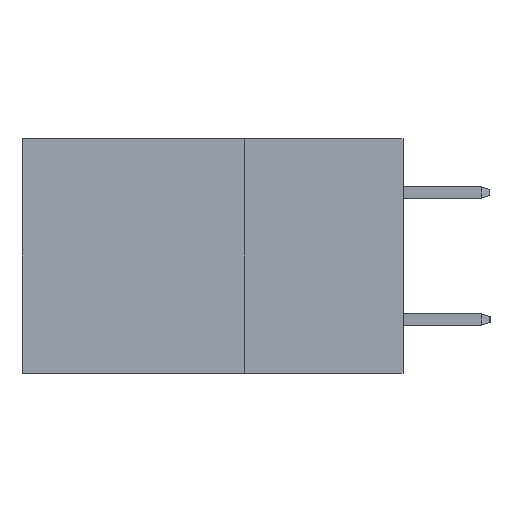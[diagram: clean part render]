
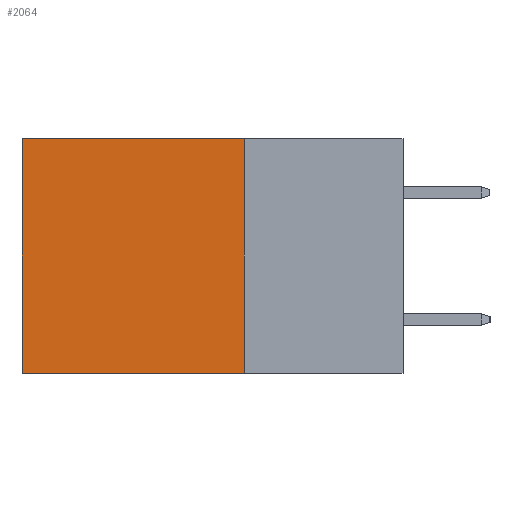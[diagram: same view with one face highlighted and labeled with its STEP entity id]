
A CAD part, left-side view. The second image highlights one B-rep face of the part: STEP entity #2064.
In plain terms, the highlighted planar face has unit normal (-1, 0, 0).
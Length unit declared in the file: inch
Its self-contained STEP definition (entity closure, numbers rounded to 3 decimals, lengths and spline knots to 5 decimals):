
#344 = EDGE_LOOP ( 'NONE', ( #1221, #7622, #7802, #9576 ) ) ;
#470 = CARTESIAN_POINT ( 'NONE',  ( 0.2875, 0.6, 0. ) ) ;
#639 = EDGE_CURVE ( 'NONE', #9602, #7751, #3348, .T. ) ;
#837 = DIRECTION ( 'NONE',  ( 0., 0., -1. ) ) ;
#1079 = CARTESIAN_POINT ( 'NONE',  ( 0.2875, 0.25, -0.37 ) ) ;
#1161 = DIRECTION ( 'NONE',  ( 0., 0., -1. ) ) ;
#1221 = ORIENTED_EDGE ( 'NONE', *, *, #9392, .T. ) ;
#1525 = VECTOR ( 'NONE', #5186, 39.37008 ) ;
#2064 = ADVANCED_FACE ( 'NONE', ( #2934 ), #4548, .F. ) ;
#2211 = CARTESIAN_POINT ( 'NONE',  ( 0.2875, 0.25, 0. ) ) ;
#2638 = LINE ( 'NONE', #470, #8165 ) ;
#2934 = FACE_OUTER_BOUND ( 'NONE', #344, .T. ) ;
#3348 = LINE ( 'NONE', #9631, #1525 ) ;
#3758 = DIRECTION ( 'NONE',  ( 1., 0., 0. ) ) ;
#3891 = VERTEX_POINT ( 'NONE', #7352 ) ;
#3948 = LINE ( 'NONE', #4538, #5496 ) ;
#4218 = CARTESIAN_POINT ( 'NONE',  ( 0.2875, 0.6, -0.37 ) ) ;
#4538 = CARTESIAN_POINT ( 'NONE',  ( 0.2875, 0.25, -0.37 ) ) ;
#4548 = PLANE ( 'NONE',  #8365 ) ;
#4951 = CARTESIAN_POINT ( 'NONE',  ( 0.2875, 0.25, 0. ) ) ;
#5186 = DIRECTION ( 'NONE',  ( 0., 0., -1. ) ) ;
#5496 = VECTOR ( 'NONE', #7556, 39.37008 ) ;
#5658 = VERTEX_POINT ( 'NONE', #4218 ) ;
#5986 = EDGE_CURVE ( 'NONE', #9602, #3891, #8708, .T. ) ;
#7352 = CARTESIAN_POINT ( 'NONE',  ( 0.2875, 0.6, 0. ) ) ;
#7556 = DIRECTION ( 'NONE',  ( 0., 1., 0. ) ) ;
#7557 = VECTOR ( 'NONE', #9489, 39.37008 ) ;
#7622 = ORIENTED_EDGE ( 'NONE', *, *, #7631, .F. ) ;
#7631 = EDGE_CURVE ( 'NONE', #7751, #5658, #3948, .T. ) ;
#7751 = VERTEX_POINT ( 'NONE', #1079 ) ;
#7802 = ORIENTED_EDGE ( 'NONE', *, *, #639, .F. ) ;
#7982 = CARTESIAN_POINT ( 'NONE',  ( 0.2875, 0.25, 0. ) ) ;
#8165 = VECTOR ( 'NONE', #1161, 39.37008 ) ;
#8365 = AXIS2_PLACEMENT_3D ( 'NONE', #2211, #3758, #837 ) ;
#8708 = LINE ( 'NONE', #4951, #7557 ) ;
#9392 = EDGE_CURVE ( 'NONE', #3891, #5658, #2638, .T. ) ;
#9489 = DIRECTION ( 'NONE',  ( 0., 1., 0. ) ) ;
#9576 = ORIENTED_EDGE ( 'NONE', *, *, #5986, .T. ) ;
#9602 = VERTEX_POINT ( 'NONE', #7982 ) ;
#9631 = CARTESIAN_POINT ( 'NONE',  ( 0.2875, 0.25, 0. ) ) ;
